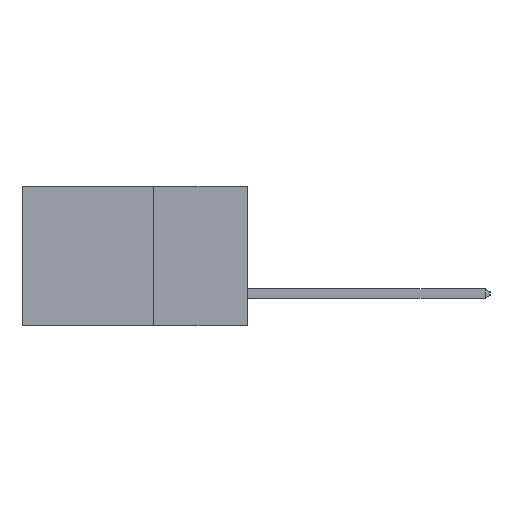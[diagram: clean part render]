
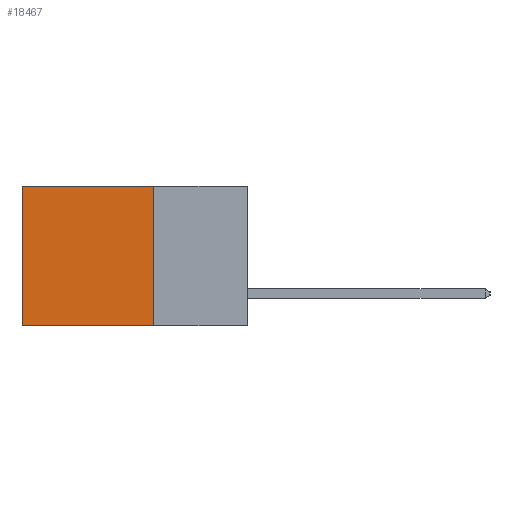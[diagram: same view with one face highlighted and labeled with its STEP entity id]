
A CAD part, left-side view. The second image highlights one B-rep face of the part: STEP entity #18467.
In plain terms, the highlighted planar face has unit normal (-1, 0, 0).
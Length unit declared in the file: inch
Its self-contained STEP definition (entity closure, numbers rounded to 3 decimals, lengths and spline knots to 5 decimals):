
#736 = AXIS2_PLACEMENT_3D ( 'NONE', #6468, #20260, #8483 ) ;
#1110 = EDGE_LOOP ( 'NONE', ( #9060, #13278, #3191, #2307 ) ) ;
#1993 = CARTESIAN_POINT ( 'NONE',  ( 0.298, 0.6, 0. ) ) ;
#2229 = EDGE_CURVE ( 'NONE', #9585, #3205, #24335, .T. ) ;
#2307 = ORIENTED_EDGE ( 'NONE', *, *, #19109, .T. ) ;
#3191 = ORIENTED_EDGE ( 'NONE', *, *, #2229, .F. ) ;
#3205 = VERTEX_POINT ( 'NONE', #16009 ) ;
#3406 = LINE ( 'NONE', #21723, #23156 ) ;
#5586 = DIRECTION ( 'NONE',  ( 0., 1., 0. ) ) ;
#6468 = CARTESIAN_POINT ( 'NONE',  ( 0.298, 0.25, 0. ) ) ;
#8483 = DIRECTION ( 'NONE',  ( 0., 0., -1. ) ) ;
#9031 = VERTEX_POINT ( 'NONE', #9467 ) ;
#9060 = ORIENTED_EDGE ( 'NONE', *, *, #15122, .T. ) ;
#9467 = CARTESIAN_POINT ( 'NONE',  ( 0.298, 0.6, -0.37 ) ) ;
#9585 = VERTEX_POINT ( 'NONE', #21003 ) ;
#9935 = DIRECTION ( 'NONE',  ( 0., 1., 0. ) ) ;
#11405 = VECTOR ( 'NONE', #9935, 39.37008 ) ;
#12014 = DIRECTION ( 'NONE',  ( 0., 0., -1. ) ) ;
#12025 = LINE ( 'NONE', #23559, #11405 ) ;
#12275 = EDGE_CURVE ( 'NONE', #3205, #9031, #17633, .T. ) ;
#12483 = VERTEX_POINT ( 'NONE', #1993 ) ;
#13278 = ORIENTED_EDGE ( 'NONE', *, *, #12275, .F. ) ;
#14370 = PLANE ( 'NONE',  #736 ) ;
#15122 = EDGE_CURVE ( 'NONE', #12483, #9031, #3406, .T. ) ;
#16009 = CARTESIAN_POINT ( 'NONE',  ( 0.298, 0.25, -0.37 ) ) ;
#17438 = CARTESIAN_POINT ( 'NONE',  ( 0.298, 0.25, -0.37 ) ) ;
#17633 = LINE ( 'NONE', #17438, #22733 ) ;
#18467 = ADVANCED_FACE ( 'NONE', ( #23313 ), #14370, .F. ) ;
#18631 = VECTOR ( 'NONE', #23507, 39.37008 ) ;
#19109 = EDGE_CURVE ( 'NONE', #9585, #12483, #12025, .T. ) ;
#20260 = DIRECTION ( 'NONE',  ( 1., 0., 0. ) ) ;
#21003 = CARTESIAN_POINT ( 'NONE',  ( 0.298, 0.25, 0. ) ) ;
#21723 = CARTESIAN_POINT ( 'NONE',  ( 0.298, 0.6, 0. ) ) ;
#22733 = VECTOR ( 'NONE', #5586, 39.37008 ) ;
#23156 = VECTOR ( 'NONE', #12014, 39.37008 ) ;
#23313 = FACE_OUTER_BOUND ( 'NONE', #1110, .T. ) ;
#23480 = CARTESIAN_POINT ( 'NONE',  ( 0.298, 0.25, 0. ) ) ;
#23507 = DIRECTION ( 'NONE',  ( 0., 0., -1. ) ) ;
#23559 = CARTESIAN_POINT ( 'NONE',  ( 0.298, 0.25, 0. ) ) ;
#24335 = LINE ( 'NONE', #23480, #18631 ) ;
